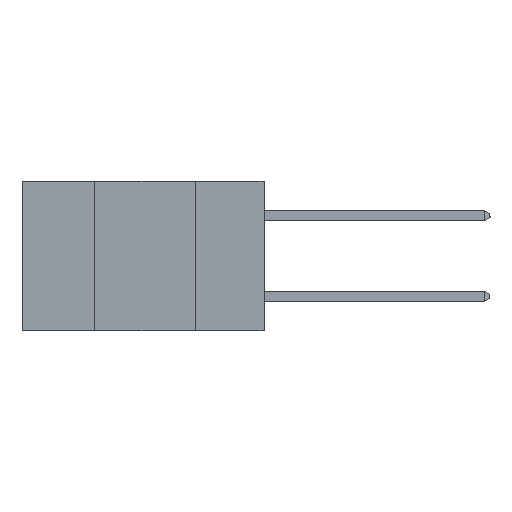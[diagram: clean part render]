
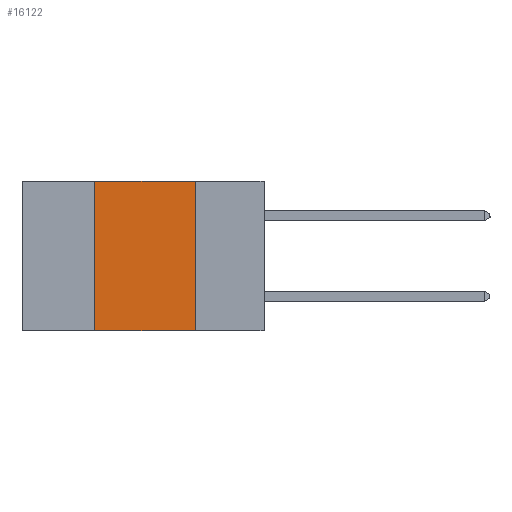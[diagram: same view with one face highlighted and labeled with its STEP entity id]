
A CAD part, left-side view. The second image highlights one B-rep face of the part: STEP entity #16122.
In plain terms, the highlighted planar face has unit normal (-1, 0, 0).
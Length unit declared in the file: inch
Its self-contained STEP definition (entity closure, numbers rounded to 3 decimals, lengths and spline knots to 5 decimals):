
#392 = FACE_OUTER_BOUND ( 'NONE', #13093, .T. ) ;
#919 = VECTOR ( 'NONE', #7921, 39.37008 ) ;
#997 = EDGE_CURVE ( 'NONE', #17028, #2060, #2268, .T. ) ;
#1024 = DIRECTION ( 'NONE',  ( 0., 0., 1. ) ) ;
#1234 = CARTESIAN_POINT ( 'NONE',  ( 0., 0.17, 0. ) ) ;
#1448 = LINE ( 'NONE', #1234, #919 ) ;
#1666 = DIRECTION ( 'NONE',  ( 1., 0., 0. ) ) ;
#2060 = VERTEX_POINT ( 'NONE', #5027 ) ;
#2268 = LINE ( 'NONE', #16387, #19097 ) ;
#2357 = ORIENTED_EDGE ( 'NONE', *, *, #20982, .F. ) ;
#2383 = CARTESIAN_POINT ( 'NONE',  ( 0., 0.17, 0. ) ) ;
#2568 = VECTOR ( 'NONE', #1024, 39.37008 ) ;
#2639 = CARTESIAN_POINT ( 'NONE',  ( 0., 0.42, 0. ) ) ;
#3451 = CARTESIAN_POINT ( 'NONE',  ( 0., 0.42, 0. ) ) ;
#4160 = LINE ( 'NONE', #4325, #15254 ) ;
#4325 = CARTESIAN_POINT ( 'NONE',  ( 0., 0.6, 0. ) ) ;
#5027 = CARTESIAN_POINT ( 'NONE',  ( 0., 0.17, -0.37 ) ) ;
#7501 = AXIS2_PLACEMENT_3D ( 'NONE', #17156, #1666, #13252 ) ;
#7525 = LINE ( 'NONE', #2639, #2568 ) ;
#7921 = DIRECTION ( 'NONE',  ( 0., 0., -1. ) ) ;
#10190 = ORIENTED_EDGE ( 'NONE', *, *, #14656, .F. ) ;
#10636 = VERTEX_POINT ( 'NONE', #3451 ) ;
#12166 = CARTESIAN_POINT ( 'NONE',  ( 0., 0.42, -0.37 ) ) ;
#13093 = EDGE_LOOP ( 'NONE', ( #10190, #2357, #17728, #13477 ) ) ;
#13252 = DIRECTION ( 'NONE',  ( 0., 0., -1. ) ) ;
#13477 = ORIENTED_EDGE ( 'NONE', *, *, #997, .T. ) ;
#14656 = EDGE_CURVE ( 'NONE', #16409, #2060, #1448, .T. ) ;
#15254 = VECTOR ( 'NONE', #17408, 39.37008 ) ;
#16122 = ADVANCED_FACE ( 'NONE', ( #392 ), #19542, .F. ) ;
#16338 = DIRECTION ( 'NONE',  ( 0., -1., 0. ) ) ;
#16387 = CARTESIAN_POINT ( 'NONE',  ( 0., 0.6, -0.37 ) ) ;
#16409 = VERTEX_POINT ( 'NONE', #2383 ) ;
#17028 = VERTEX_POINT ( 'NONE', #12166 ) ;
#17156 = CARTESIAN_POINT ( 'NONE',  ( 0., 0.6, 0. ) ) ;
#17408 = DIRECTION ( 'NONE',  ( 0., -1., 0. ) ) ;
#17728 = ORIENTED_EDGE ( 'NONE', *, *, #21011, .F. ) ;
#19097 = VECTOR ( 'NONE', #16338, 39.37008 ) ;
#19542 = PLANE ( 'NONE',  #7501 ) ;
#20982 = EDGE_CURVE ( 'NONE', #10636, #16409, #4160, .T. ) ;
#21011 = EDGE_CURVE ( 'NONE', #17028, #10636, #7525, .T. ) ;
